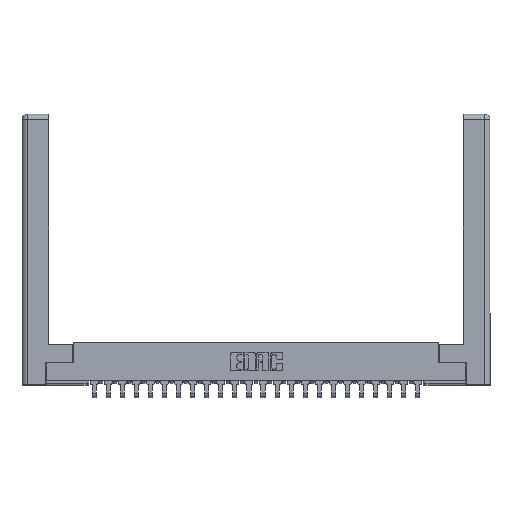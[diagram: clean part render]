
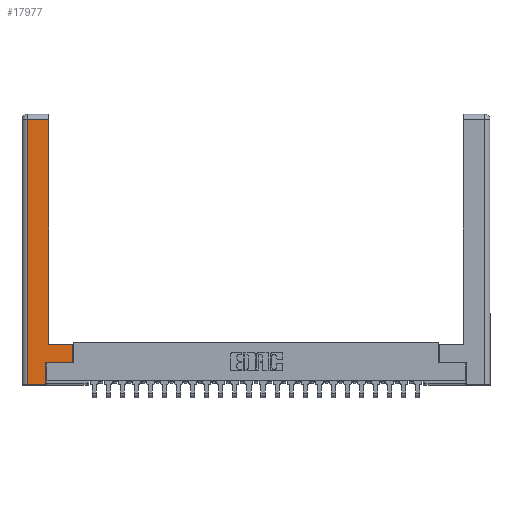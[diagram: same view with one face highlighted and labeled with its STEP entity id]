
A CAD part, top view. The second image highlights one B-rep face of the part: STEP entity #17977.
In plain terms, the highlighted planar face has unit normal (0, 0, 1).
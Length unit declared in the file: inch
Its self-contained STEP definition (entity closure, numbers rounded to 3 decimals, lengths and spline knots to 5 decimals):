
#217 = DIRECTION ( 'NONE',  ( -1., 0., 0. ) ) ;
#278 = CARTESIAN_POINT ( 'NONE',  ( 0.295, 3., 0. ) ) ;
#468 = FACE_OUTER_BOUND ( 'NONE', #11048, .T. ) ;
#1210 = ORIENTED_EDGE ( 'NONE', *, *, #2246, .T. ) ;
#1680 = CARTESIAN_POINT ( 'NONE',  ( 0.565, 0.245, 0. ) ) ;
#1769 = ORIENTED_EDGE ( 'NONE', *, *, #21431, .T. ) ;
#2010 = CARTESIAN_POINT ( 'NONE',  ( 0.565, 0.45, 0. ) ) ;
#2161 = DIRECTION ( 'NONE',  ( -1., 0., 0. ) ) ;
#2246 = EDGE_CURVE ( 'NONE', #4858, #6859, #4130, .T. ) ;
#2356 = EDGE_CURVE ( 'NONE', #14539, #4858, #19801, .T. ) ;
#3054 = VERTEX_POINT ( 'NONE', #5229 ) ;
#3917 = CARTESIAN_POINT ( 'NONE',  ( 0., 0., 0. ) ) ;
#3976 = VERTEX_POINT ( 'NONE', #15920 ) ;
#3993 = VECTOR ( 'NONE', #7481, 39.37008 ) ;
#4130 = LINE ( 'NONE', #12791, #6887 ) ;
#4706 = CARTESIAN_POINT ( 'NONE',  ( 0.0615, 2.94, 0. ) ) ;
#4858 = VERTEX_POINT ( 'NONE', #2010 ) ;
#4974 = VERTEX_POINT ( 'NONE', #15405 ) ;
#5229 = CARTESIAN_POINT ( 'NONE',  ( 0.295, 2.94, 0. ) ) ;
#5263 = ORIENTED_EDGE ( 'NONE', *, *, #10695, .T. ) ;
#5271 = AXIS2_PLACEMENT_3D ( 'NONE', #3917, #11911, #2161 ) ;
#5922 = VERTEX_POINT ( 'NONE', #10764 ) ;
#6344 = LINE ( 'NONE', #20621, #23256 ) ;
#6476 = DIRECTION ( 'NONE',  ( 0., -1., 0. ) ) ;
#6859 = VERTEX_POINT ( 'NONE', #21878 ) ;
#6887 = VECTOR ( 'NONE', #8856, 39.37008 ) ;
#6889 = DIRECTION ( 'NONE',  ( 0., 1., 0. ) ) ;
#7081 = VECTOR ( 'NONE', #10094, 39.37008 ) ;
#7234 = LINE ( 'NONE', #20361, #10603 ) ;
#7481 = DIRECTION ( 'NONE',  ( 1., 0., 0. ) ) ;
#8550 = EDGE_CURVE ( 'NONE', #5922, #4974, #6344, .T. ) ;
#8694 = CARTESIAN_POINT ( 'NONE',  ( 0.565, 0.45, 0. ) ) ;
#8856 = DIRECTION ( 'NONE',  ( -1., 0., 0. ) ) ;
#8970 = ORIENTED_EDGE ( 'NONE', *, *, #2356, .T. ) ;
#10094 = DIRECTION ( 'NONE',  ( 0., 1., 0. ) ) ;
#10603 = VECTOR ( 'NONE', #6476, 39.37008 ) ;
#10695 = EDGE_CURVE ( 'NONE', #3976, #14539, #21196, .T. ) ;
#10764 = CARTESIAN_POINT ( 'NONE',  ( 0.0615, 0., 0. ) ) ;
#11048 = EDGE_LOOP ( 'NONE', ( #1769, #23145, #22386, #19064, #17696, #5263, #8970, #1210 ) ) ;
#11911 = DIRECTION ( 'NONE',  ( 0., 0., -1. ) ) ;
#12053 = CARTESIAN_POINT ( 'NONE',  ( 0.265, 0.245, 0. ) ) ;
#12704 = CARTESIAN_POINT ( 'NONE',  ( 0.0615, 2.94, 0. ) ) ;
#12791 = CARTESIAN_POINT ( 'NONE',  ( 0.295, 0.45, 0. ) ) ;
#14531 = VECTOR ( 'NONE', #6889, 39.37008 ) ;
#14539 = VERTEX_POINT ( 'NONE', #21325 ) ;
#14988 = DIRECTION ( 'NONE',  ( 1., 0., 0. ) ) ;
#15405 = CARTESIAN_POINT ( 'NONE',  ( 0.265, 0., 0. ) ) ;
#15446 = VECTOR ( 'NONE', #217, 39.37008 ) ;
#15920 = CARTESIAN_POINT ( 'NONE',  ( 0.265, 0.245, 0. ) ) ;
#16665 = VERTEX_POINT ( 'NONE', #12704 ) ;
#17411 = VECTOR ( 'NONE', #21727, 39.37008 ) ;
#17696 = ORIENTED_EDGE ( 'NONE', *, *, #22179, .T. ) ;
#17977 = ADVANCED_FACE ( 'NONE', ( #468 ), #19807, .F. ) ;
#18657 = LINE ( 'NONE', #278, #17411 ) ;
#18728 = LINE ( 'NONE', #12053, #7081 ) ;
#18825 = EDGE_CURVE ( 'NONE', #16665, #5922, #7234, .T. ) ;
#19064 = ORIENTED_EDGE ( 'NONE', *, *, #8550, .T. ) ;
#19454 = EDGE_CURVE ( 'NONE', #3054, #16665, #22252, .T. ) ;
#19801 = LINE ( 'NONE', #8694, #14531 ) ;
#19807 = PLANE ( 'NONE',  #5271 ) ;
#20361 = CARTESIAN_POINT ( 'NONE',  ( 0.0615, 0., 0. ) ) ;
#20621 = CARTESIAN_POINT ( 'NONE',  ( 0.265, 0., 0. ) ) ;
#21196 = LINE ( 'NONE', #1680, #3993 ) ;
#21325 = CARTESIAN_POINT ( 'NONE',  ( 0.565, 0.245, 0. ) ) ;
#21431 = EDGE_CURVE ( 'NONE', #6859, #3054, #18657, .T. ) ;
#21727 = DIRECTION ( 'NONE',  ( 0., 1., 0. ) ) ;
#21878 = CARTESIAN_POINT ( 'NONE',  ( 0.295, 0.45, 0. ) ) ;
#22179 = EDGE_CURVE ( 'NONE', #4974, #3976, #18728, .T. ) ;
#22252 = LINE ( 'NONE', #4706, #15446 ) ;
#22386 = ORIENTED_EDGE ( 'NONE', *, *, #18825, .T. ) ;
#23145 = ORIENTED_EDGE ( 'NONE', *, *, #19454, .T. ) ;
#23256 = VECTOR ( 'NONE', #14988, 39.37008 ) ;
